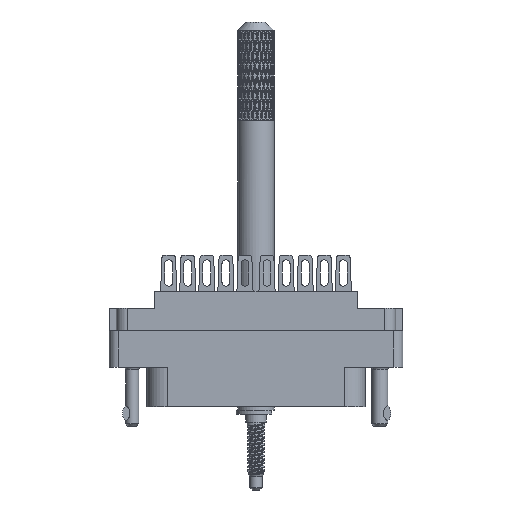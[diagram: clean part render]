
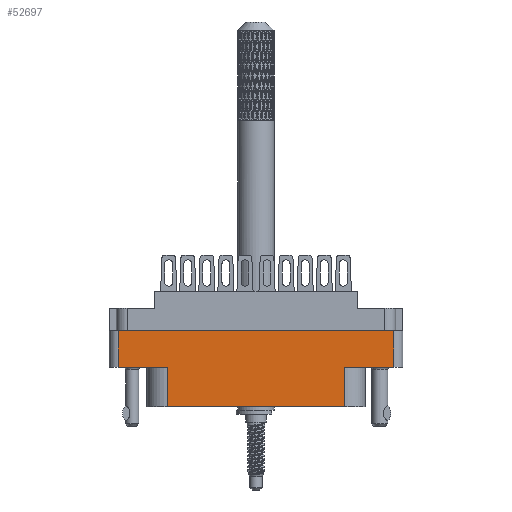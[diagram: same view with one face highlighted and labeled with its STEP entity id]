
A CAD part, front view. The second image highlights one B-rep face of the part: STEP entity #52697.
In plain terms, the highlighted planar face has unit normal (0, -1, 0).
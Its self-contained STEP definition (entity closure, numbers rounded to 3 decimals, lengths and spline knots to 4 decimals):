
#1187 = EDGE_CURVE ( 'NONE', #24223, #45060, #38067, .T. ) ;
#1988 = EDGE_CURVE ( 'NONE', #31987, #24223, #16248, .T. ) ;
#3855 = EDGE_CURVE ( 'NONE', #43109, #31987, #97807, .T. ) ;
#3886 = EDGE_CURVE ( 'NONE', #102332, #43109, #109930, .T. ) ;
#4428 = DIRECTION ( 'NONE',  ( 1., 0., 0. ) ) ;
#5287 = ORIENTED_EDGE ( 'NONE', *, *, #111964, .T. ) ;
#7120 = CARTESIAN_POINT ( 'NONE',  ( 0.604, -0.438, -0.52 ) ) ;
#8217 = DIRECTION ( 'NONE',  ( 0., 0., 1. ) ) ;
#11894 = VECTOR ( 'NONE', #34830, 39.3701 ) ;
#15805 = CARTESIAN_POINT ( 'NONE',  ( 0.938, -0.438, -0.268 ) ) ;
#15956 = DIRECTION ( 'NONE',  ( 0., 0., -1. ) ) ;
#16248 = LINE ( 'NONE', #20976, #106215 ) ;
#17653 = DIRECTION ( 'NONE',  ( 1., 0., 0. ) ) ;
#20976 = CARTESIAN_POINT ( 'NONE',  ( -0.604, -0.438, -0.789 ) ) ;
#22335 = DIRECTION ( 'NONE',  ( 0., 0., -1. ) ) ;
#24223 = VERTEX_POINT ( 'NONE', #72028 ) ;
#31987 = VERTEX_POINT ( 'NONE', #48178 ) ;
#32384 = ORIENTED_EDGE ( 'NONE', *, *, #1187, .T. ) ;
#34054 = CARTESIAN_POINT ( 'NONE',  ( -1., -0.438, -0.789 ) ) ;
#34830 = DIRECTION ( 'NONE',  ( 0., 0., 1. ) ) ;
#34973 = DIRECTION ( 'NONE',  ( 0., -1., 0. ) ) ;
#35016 = LINE ( 'NONE', #96132, #11894 ) ;
#37122 = VERTEX_POINT ( 'NONE', #75476 ) ;
#38067 = LINE ( 'NONE', #34054, #74962 ) ;
#39665 = ORIENTED_EDGE ( 'NONE', *, *, #1988, .T. ) ;
#40940 = DIRECTION ( 'NONE',  ( -1., 0., 0. ) ) ;
#41679 = ORIENTED_EDGE ( 'NONE', *, *, #58397, .F. ) ;
#42756 = EDGE_CURVE ( 'NONE', #45060, #37122, #73310, .T. ) ;
#43109 = VERTEX_POINT ( 'NONE', #90409 ) ;
#43132 = VECTOR ( 'NONE', #22335, 39.3701 ) ;
#44807 = VERTEX_POINT ( 'NONE', #15805 ) ;
#45060 = VERTEX_POINT ( 'NONE', #56039 ) ;
#45071 = CARTESIAN_POINT ( 'NONE',  ( -0.938, -0.438, -0.268 ) ) ;
#45862 = EDGE_CURVE ( 'NONE', #85472, #37122, #62594, .T. ) ;
#46740 = ORIENTED_EDGE ( 'NONE', *, *, #45862, .F. ) ;
#48178 = CARTESIAN_POINT ( 'NONE',  ( -0.604, -0.438, -0.52 ) ) ;
#49274 = CARTESIAN_POINT ( 'NONE',  ( 0., -0.438, -0.52 ) ) ;
#50103 = CARTESIAN_POINT ( 'NONE',  ( 0., -0.438, -0.52 ) ) ;
#51925 = DIRECTION ( 'NONE',  ( 1., 0., 0. ) ) ;
#52697 = ADVANCED_FACE ( 'NONE', ( #60210 ), #68131, .T. ) ;
#56039 = CARTESIAN_POINT ( 'NONE',  ( 0.604, -0.438, -0.789 ) ) ;
#57296 = EDGE_LOOP ( 'NONE', ( #41679, #99239, #63938, #39665, #32384, #72237, #46740, #5287 ) ) ;
#58397 = EDGE_CURVE ( 'NONE', #102332, #44807, #98596, .T. ) ;
#59628 = VECTOR ( 'NONE', #8217, 39.3701 ) ;
#60210 = FACE_OUTER_BOUND ( 'NONE', #57296, .T. ) ;
#60475 = CARTESIAN_POINT ( 'NONE',  ( 0.938, -0.438, -0.52 ) ) ;
#62594 = LINE ( 'NONE', #50103, #85808 ) ;
#63938 = ORIENTED_EDGE ( 'NONE', *, *, #3855, .T. ) ;
#68131 = PLANE ( 'NONE',  #94538 ) ;
#72028 = CARTESIAN_POINT ( 'NONE',  ( -0.604, -0.438, -0.789 ) ) ;
#72237 = ORIENTED_EDGE ( 'NONE', *, *, #42756, .T. ) ;
#73310 = LINE ( 'NONE', #7120, #59628 ) ;
#74962 = VECTOR ( 'NONE', #17653, 39.3701 ) ;
#75476 = CARTESIAN_POINT ( 'NONE',  ( 0.604, -0.438, -0.52 ) ) ;
#84036 = VECTOR ( 'NONE', #4428, 39.3701 ) ;
#85472 = VERTEX_POINT ( 'NONE', #60475 ) ;
#85808 = VECTOR ( 'NONE', #40940, 39.3701 ) ;
#87226 = CARTESIAN_POINT ( 'NONE',  ( -1., -0.438, -0.789 ) ) ;
#90409 = CARTESIAN_POINT ( 'NONE',  ( -0.938, -0.438, -0.52 ) ) ;
#94538 = AXIS2_PLACEMENT_3D ( 'NONE', #87226, #34973, #15956 ) ;
#96132 = CARTESIAN_POINT ( 'NONE',  ( 0.938, -0.438, -0.789 ) ) ;
#97807 = LINE ( 'NONE', #49274, #84036 ) ;
#98596 = LINE ( 'NONE', #103409, #102674 ) ;
#99239 = ORIENTED_EDGE ( 'NONE', *, *, #3886, .T. ) ;
#102332 = VERTEX_POINT ( 'NONE', #45071 ) ;
#102674 = VECTOR ( 'NONE', #51925, 39.3701 ) ;
#103409 = CARTESIAN_POINT ( 'NONE',  ( 0., -0.438, -0.268 ) ) ;
#106215 = VECTOR ( 'NONE', #106654, 39.3701 ) ;
#106654 = DIRECTION ( 'NONE',  ( 0., 0., -1. ) ) ;
#109862 = CARTESIAN_POINT ( 'NONE',  ( -0.938, -0.438, -0.789 ) ) ;
#109930 = LINE ( 'NONE', #109862, #43132 ) ;
#111964 = EDGE_CURVE ( 'NONE', #85472, #44807, #35016, .T. ) ;
